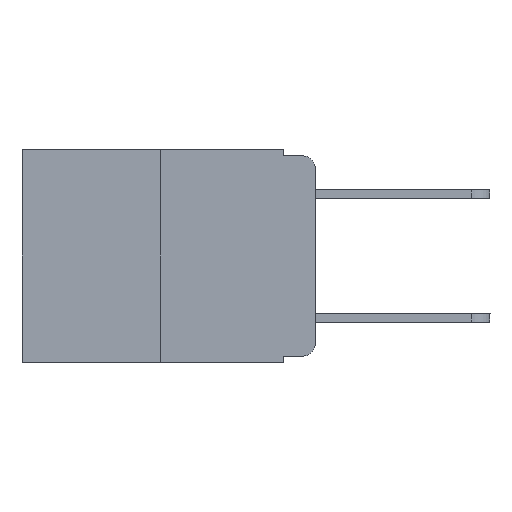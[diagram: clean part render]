
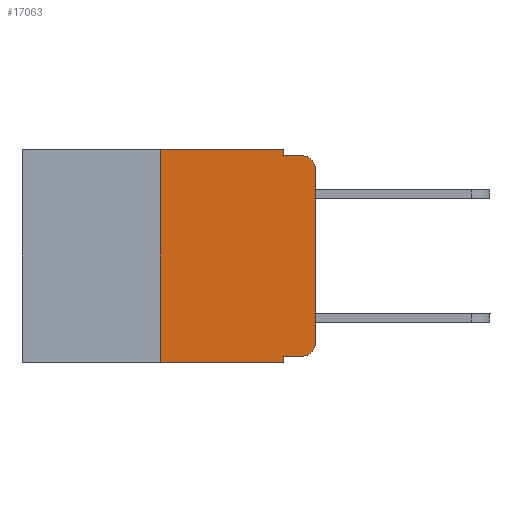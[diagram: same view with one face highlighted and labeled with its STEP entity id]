
A CAD part, left-side view. The second image highlights one B-rep face of the part: STEP entity #17063.
In plain terms, the highlighted planar face has unit normal (-1, 0, 0).
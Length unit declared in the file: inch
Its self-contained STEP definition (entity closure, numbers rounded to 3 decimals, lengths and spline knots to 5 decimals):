
#225 = CARTESIAN_POINT ( 'NONE',  ( 0., 0.02, -0.01 ) ) ;
#236 = EDGE_CURVE ( 'NONE', #13509, #4105, #3660, .T. ) ;
#303 = VERTEX_POINT ( 'NONE', #20410 ) ;
#960 = LINE ( 'NONE', #13432, #3323 ) ;
#1251 = EDGE_CURVE ( 'NONE', #13509, #5883, #2554, .T. ) ;
#1442 = EDGE_CURVE ( 'NONE', #303, #17563, #16374, .T. ) ;
#1701 = VERTEX_POINT ( 'NONE', #13540 ) ;
#1744 = DIRECTION ( 'NONE',  ( 0., -1., 0. ) ) ;
#1921 = CARTESIAN_POINT ( 'NONE',  ( 0., 0.051, 0. ) ) ;
#2063 = VERTEX_POINT ( 'NONE', #16475 ) ;
#2405 = VECTOR ( 'NONE', #9010, 39.37008 ) ;
#2413 = CARTESIAN_POINT ( 'NONE',  ( 0., 0.25, 0. ) ) ;
#2477 = DIRECTION ( 'NONE',  ( 0., 0., 1. ) ) ;
#2554 = LINE ( 'NONE', #1921, #8301 ) ;
#3163 = AXIS2_PLACEMENT_3D ( 'NONE', #18567, #3262, #3984 ) ;
#3262 = DIRECTION ( 'NONE',  ( -1., 0., 0. ) ) ;
#3323 = VECTOR ( 'NONE', #20096, 39.37008 ) ;
#3660 = LINE ( 'NONE', #14645, #18809 ) ;
#3974 = VERTEX_POINT ( 'NONE', #225 ) ;
#3984 = DIRECTION ( 'NONE',  ( 0., 0., -1. ) ) ;
#4105 = VERTEX_POINT ( 'NONE', #17031 ) ;
#4287 = ORIENTED_EDGE ( 'NONE', *, *, #236, .T. ) ;
#4555 = ORIENTED_EDGE ( 'NONE', *, *, #7299, .T. ) ;
#4580 = VECTOR ( 'NONE', #1744, 39.37008 ) ;
#5691 = CARTESIAN_POINT ( 'NONE',  ( 0., 0.473, -0.343 ) ) ;
#5883 = VERTEX_POINT ( 'NONE', #19374 ) ;
#5919 = EDGE_CURVE ( 'NONE', #4105, #1701, #17352, .T. ) ;
#6299 = EDGE_LOOP ( 'NONE', ( #4555, #17917, #21482, #21300, #9760, #20971, #13362, #11555, #4287, #18682 ) ) ;
#7299 = EDGE_CURVE ( 'NONE', #1701, #12829, #11807, .T. ) ;
#7671 = AXIS2_PLACEMENT_3D ( 'NONE', #18737, #12083, #11929 ) ;
#7947 = AXIS2_PLACEMENT_3D ( 'NONE', #9543, #17877, #8019 ) ;
#8019 = DIRECTION ( 'NONE',  ( 0., 0., -1. ) ) ;
#8255 = DIRECTION ( 'NONE',  ( 0., 0., -1. ) ) ;
#8301 = VECTOR ( 'NONE', #15276, 39.37008 ) ;
#9006 = LINE ( 'NONE', #16639, #4580 ) ;
#9010 = DIRECTION ( 'NONE',  ( 0., -1., 0. ) ) ;
#9084 = VECTOR ( 'NONE', #2477, 39.37008 ) ;
#9370 = CARTESIAN_POINT ( 'NONE',  ( 0., 0., 0. ) ) ;
#9543 = CARTESIAN_POINT ( 'NONE',  ( 0., 0.473, 0. ) ) ;
#9760 = ORIENTED_EDGE ( 'NONE', *, *, #13455, .F. ) ;
#10543 = CARTESIAN_POINT ( 'NONE',  ( 0., 0.25, 0. ) ) ;
#11136 = EDGE_CURVE ( 'NONE', #303, #5883, #12063, .T. ) ;
#11440 = CARTESIAN_POINT ( 'NONE',  ( 0., 0.051, 0. ) ) ;
#11555 = ORIENTED_EDGE ( 'NONE', *, *, #1251, .F. ) ;
#11807 = LINE ( 'NONE', #9370, #12091 ) ;
#11929 = DIRECTION ( 'NONE',  ( 0., 0., -1. ) ) ;
#12063 = LINE ( 'NONE', #5691, #2405 ) ;
#12083 = DIRECTION ( 'NONE',  ( -1., 0., 0. ) ) ;
#12091 = VECTOR ( 'NONE', #21080, 39.37008 ) ;
#12490 = VECTOR ( 'NONE', #8255, 39.37008 ) ;
#12528 = CARTESIAN_POINT ( 'NONE',  ( 0., 0.051, -0.333 ) ) ;
#12829 = VERTEX_POINT ( 'NONE', #21571 ) ;
#13360 = EDGE_CURVE ( 'NONE', #14814, #2063, #20872, .T. ) ;
#13362 = ORIENTED_EDGE ( 'NONE', *, *, #11136, .T. ) ;
#13432 = CARTESIAN_POINT ( 'NONE',  ( 0., 0.473, 0. ) ) ;
#13455 = EDGE_CURVE ( 'NONE', #17563, #14814, #960, .T. ) ;
#13509 = VERTEX_POINT ( 'NONE', #12528 ) ;
#13540 = CARTESIAN_POINT ( 'NONE',  ( 0., 0., -0.313 ) ) ;
#13987 = CARTESIAN_POINT ( 'NONE',  ( 0., 0.051, 0. ) ) ;
#14645 = CARTESIAN_POINT ( 'NONE',  ( 0., 0.051, -0.333 ) ) ;
#14814 = VERTEX_POINT ( 'NONE', #13987 ) ;
#15276 = DIRECTION ( 'NONE',  ( 0., 0., -1. ) ) ;
#16114 = PLANE ( 'NONE',  #7947 ) ;
#16374 = LINE ( 'NONE', #2413, #9084 ) ;
#16475 = CARTESIAN_POINT ( 'NONE',  ( 0., 0.051, -0.01 ) ) ;
#16520 = EDGE_CURVE ( 'NONE', #12829, #3974, #17252, .T. ) ;
#16639 = CARTESIAN_POINT ( 'NONE',  ( 0., 0.051, -0.01 ) ) ;
#17031 = CARTESIAN_POINT ( 'NONE',  ( 0., 0.02, -0.333 ) ) ;
#17063 = ADVANCED_FACE ( 'NONE', ( #18792 ), #16114, .F. ) ;
#17252 = CIRCLE ( 'NONE', #7671, 0.02 ) ;
#17352 = CIRCLE ( 'NONE', #3163, 0.02 ) ;
#17563 = VERTEX_POINT ( 'NONE', #10543 ) ;
#17877 = DIRECTION ( 'NONE',  ( 1., 0., 0. ) ) ;
#17881 = DIRECTION ( 'NONE',  ( 0., -1., 0. ) ) ;
#17917 = ORIENTED_EDGE ( 'NONE', *, *, #16520, .T. ) ;
#18567 = CARTESIAN_POINT ( 'NONE',  ( 0., 0.02, -0.313 ) ) ;
#18682 = ORIENTED_EDGE ( 'NONE', *, *, #5919, .T. ) ;
#18737 = CARTESIAN_POINT ( 'NONE',  ( 0., 0.02, -0.03 ) ) ;
#18792 = FACE_OUTER_BOUND ( 'NONE', #6299, .T. ) ;
#18809 = VECTOR ( 'NONE', #17881, 39.37008 ) ;
#19374 = CARTESIAN_POINT ( 'NONE',  ( 0., 0.051, -0.343 ) ) ;
#20096 = DIRECTION ( 'NONE',  ( 0., -1., 0. ) ) ;
#20225 = EDGE_CURVE ( 'NONE', #2063, #3974, #9006, .T. ) ;
#20410 = CARTESIAN_POINT ( 'NONE',  ( 0., 0.25, -0.343 ) ) ;
#20872 = LINE ( 'NONE', #11440, #12490 ) ;
#20971 = ORIENTED_EDGE ( 'NONE', *, *, #1442, .F. ) ;
#21080 = DIRECTION ( 'NONE',  ( 0., 0., 1. ) ) ;
#21300 = ORIENTED_EDGE ( 'NONE', *, *, #13360, .F. ) ;
#21482 = ORIENTED_EDGE ( 'NONE', *, *, #20225, .F. ) ;
#21571 = CARTESIAN_POINT ( 'NONE',  ( 0., 0., -0.03 ) ) ;
